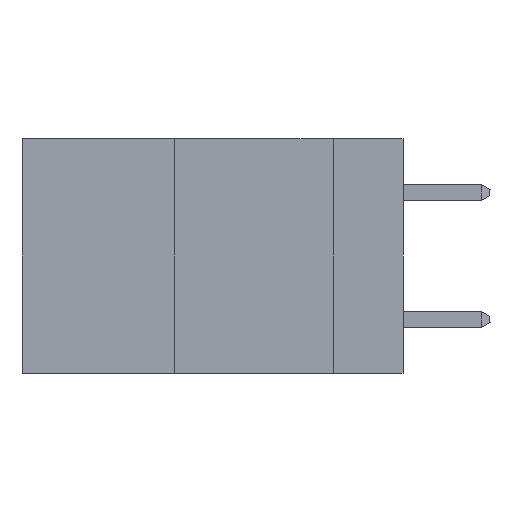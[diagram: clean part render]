
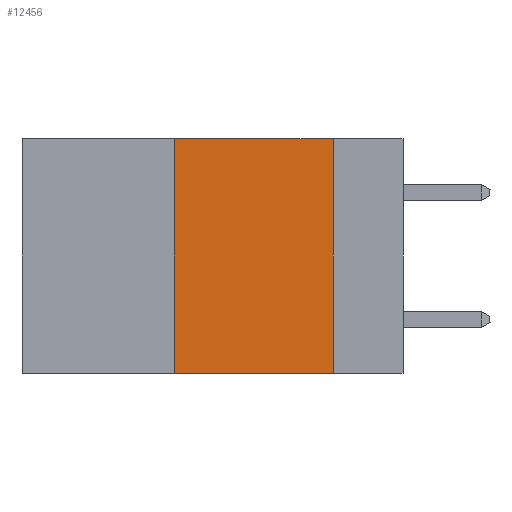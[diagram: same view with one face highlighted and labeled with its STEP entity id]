
A CAD part, left-side view. The second image highlights one B-rep face of the part: STEP entity #12456.
In plain terms, the highlighted planar face has unit normal (-1, 0, 0).
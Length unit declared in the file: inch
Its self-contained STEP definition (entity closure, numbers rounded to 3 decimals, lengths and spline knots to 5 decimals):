
#179 = CARTESIAN_POINT ( 'NONE',  ( 0., 0.36, 0. ) ) ;
#276 = DIRECTION ( 'NONE',  ( 0., 0., -1. ) ) ;
#521 = DIRECTION ( 'NONE',  ( 0., -1., 0. ) ) ;
#1766 = ORIENTED_EDGE ( 'NONE', *, *, #18982, .F. ) ;
#2951 = LINE ( 'NONE', #12450, #6390 ) ;
#3366 = VERTEX_POINT ( 'NONE', #4797 ) ;
#4370 = DIRECTION ( 'NONE',  ( 1., 0., 0. ) ) ;
#4797 = CARTESIAN_POINT ( 'NONE',  ( 0., 0.11, -0.37 ) ) ;
#4846 = LINE ( 'NONE', #20474, #10950 ) ;
#5264 = EDGE_LOOP ( 'NONE', ( #20318, #12826, #1766, #19039 ) ) ;
#5754 = VERTEX_POINT ( 'NONE', #14349 ) ;
#6390 = VECTOR ( 'NONE', #521, 39.37008 ) ;
#6510 = EDGE_CURVE ( 'NONE', #14518, #3366, #11965, .T. ) ;
#6651 = CARTESIAN_POINT ( 'NONE',  ( 0., 0.11, 0. ) ) ;
#7474 = VERTEX_POINT ( 'NONE', #6651 ) ;
#8588 = DIRECTION ( 'NONE',  ( 0., 0., 1. ) ) ;
#9443 = DIRECTION ( 'NONE',  ( 0., 0., -1. ) ) ;
#9875 = DIRECTION ( 'NONE',  ( 0., -1., 0. ) ) ;
#10950 = VECTOR ( 'NONE', #276, 39.37008 ) ;
#11965 = LINE ( 'NONE', #16807, #13049 ) ;
#12450 = CARTESIAN_POINT ( 'NONE',  ( 0., 0.6, 0. ) ) ;
#12456 = ADVANCED_FACE ( 'NONE', ( #14224 ), #19714, .F. ) ;
#12826 = ORIENTED_EDGE ( 'NONE', *, *, #20947, .F. ) ;
#13049 = VECTOR ( 'NONE', #9875, 39.37008 ) ;
#14224 = FACE_OUTER_BOUND ( 'NONE', #5264, .T. ) ;
#14349 = CARTESIAN_POINT ( 'NONE',  ( 0., 0.36, 0. ) ) ;
#14518 = VERTEX_POINT ( 'NONE', #21495 ) ;
#15804 = VECTOR ( 'NONE', #8588, 39.37008 ) ;
#16807 = CARTESIAN_POINT ( 'NONE',  ( 0., 0.6, -0.37 ) ) ;
#18982 = EDGE_CURVE ( 'NONE', #14518, #5754, #20069, .T. ) ;
#19025 = AXIS2_PLACEMENT_3D ( 'NONE', #19783, #4370, #9443 ) ;
#19039 = ORIENTED_EDGE ( 'NONE', *, *, #6510, .T. ) ;
#19714 = PLANE ( 'NONE',  #19025 ) ;
#19783 = CARTESIAN_POINT ( 'NONE',  ( 0., 0.6, 0. ) ) ;
#20069 = LINE ( 'NONE', #179, #15804 ) ;
#20266 = EDGE_CURVE ( 'NONE', #7474, #3366, #4846, .T. ) ;
#20318 = ORIENTED_EDGE ( 'NONE', *, *, #20266, .F. ) ;
#20474 = CARTESIAN_POINT ( 'NONE',  ( 0., 0.11, 0. ) ) ;
#20947 = EDGE_CURVE ( 'NONE', #5754, #7474, #2951, .T. ) ;
#21495 = CARTESIAN_POINT ( 'NONE',  ( 0., 0.36, -0.37 ) ) ;
